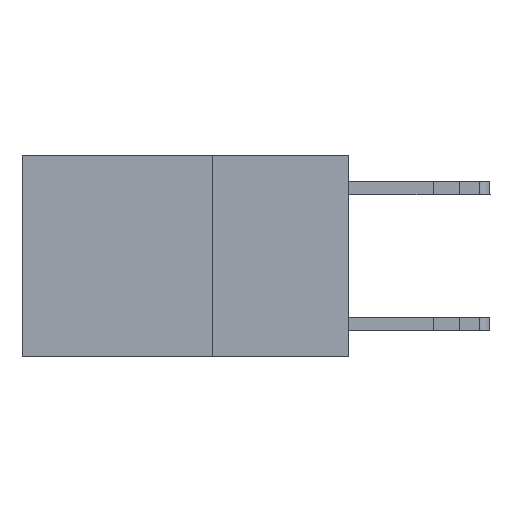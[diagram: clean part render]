
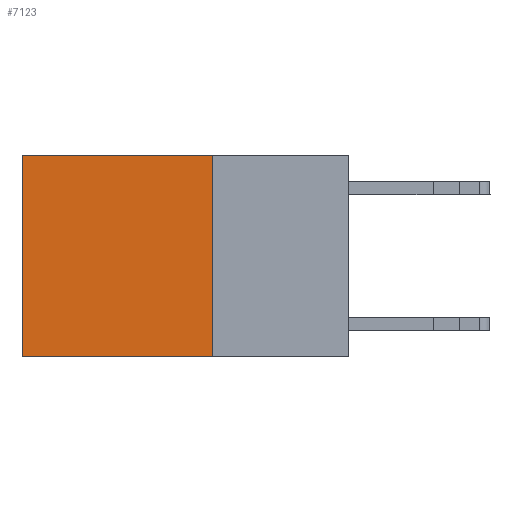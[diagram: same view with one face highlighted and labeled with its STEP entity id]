
A CAD part, left-side view. The second image highlights one B-rep face of the part: STEP entity #7123.
In plain terms, the highlighted planar face has unit normal (-1, 0, 0).
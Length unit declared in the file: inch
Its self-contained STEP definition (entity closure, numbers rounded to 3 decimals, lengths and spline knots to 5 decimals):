
#180 = EDGE_LOOP ( 'NONE', ( #11114, #5601, #3608, #8760 ) ) ;
#394 = DIRECTION ( 'NONE',  ( 0., 0., -1. ) ) ;
#402 = VECTOR ( 'NONE', #13993, 39.37008 ) ;
#458 = VECTOR ( 'NONE', #17099, 39.37008 ) ;
#1374 = DIRECTION ( 'NONE',  ( 0., 1., 0. ) ) ;
#1629 = EDGE_CURVE ( 'NONE', #11020, #14131, #5876, .T. ) ;
#2076 = VERTEX_POINT ( 'NONE', #12773 ) ;
#2091 = FACE_OUTER_BOUND ( 'NONE', #180, .T. ) ;
#3115 = VERTEX_POINT ( 'NONE', #11965 ) ;
#3248 = VECTOR ( 'NONE', #1374, 39.37008 ) ;
#3608 = ORIENTED_EDGE ( 'NONE', *, *, #1629, .F. ) ;
#3946 = CARTESIAN_POINT ( 'NONE',  ( 0.2625, 0.25, -0.37 ) ) ;
#4044 = CARTESIAN_POINT ( 'NONE',  ( 0.2625, 0.25, -0.37 ) ) ;
#4619 = VECTOR ( 'NONE', #12863, 39.37008 ) ;
#5601 = ORIENTED_EDGE ( 'NONE', *, *, #7323, .F. ) ;
#5876 = LINE ( 'NONE', #16678, #458 ) ;
#6657 = EDGE_CURVE ( 'NONE', #11020, #3115, #16741, .T. ) ;
#7123 = ADVANCED_FACE ( 'NONE', ( #2091 ), #15423, .F. ) ;
#7323 = EDGE_CURVE ( 'NONE', #14131, #2076, #10678, .T. ) ;
#7493 = CARTESIAN_POINT ( 'NONE',  ( 0.2625, 0.25, 0. ) ) ;
#7566 = EDGE_CURVE ( 'NONE', #3115, #2076, #15316, .T. ) ;
#7758 = AXIS2_PLACEMENT_3D ( 'NONE', #7493, #11308, #394 ) ;
#8551 = CARTESIAN_POINT ( 'NONE',  ( 0.2625, 0.6, 0. ) ) ;
#8760 = ORIENTED_EDGE ( 'NONE', *, *, #6657, .T. ) ;
#10678 = LINE ( 'NONE', #4044, #3248 ) ;
#11020 = VERTEX_POINT ( 'NONE', #16720 ) ;
#11114 = ORIENTED_EDGE ( 'NONE', *, *, #7566, .T. ) ;
#11308 = DIRECTION ( 'NONE',  ( 1., 0., 0. ) ) ;
#11965 = CARTESIAN_POINT ( 'NONE',  ( 0.2625, 0.6, 0. ) ) ;
#12773 = CARTESIAN_POINT ( 'NONE',  ( 0.2625, 0.6, -0.37 ) ) ;
#12863 = DIRECTION ( 'NONE',  ( 0., 1., 0. ) ) ;
#13993 = DIRECTION ( 'NONE',  ( 0., 0., -1. ) ) ;
#14131 = VERTEX_POINT ( 'NONE', #3946 ) ;
#15316 = LINE ( 'NONE', #8551, #402 ) ;
#15423 = PLANE ( 'NONE',  #7758 ) ;
#15531 = CARTESIAN_POINT ( 'NONE',  ( 0.2625, 0.25, 0. ) ) ;
#16678 = CARTESIAN_POINT ( 'NONE',  ( 0.2625, 0.25, 0. ) ) ;
#16720 = CARTESIAN_POINT ( 'NONE',  ( 0.2625, 0.25, 0. ) ) ;
#16741 = LINE ( 'NONE', #15531, #4619 ) ;
#17099 = DIRECTION ( 'NONE',  ( 0., 0., -1. ) ) ;
